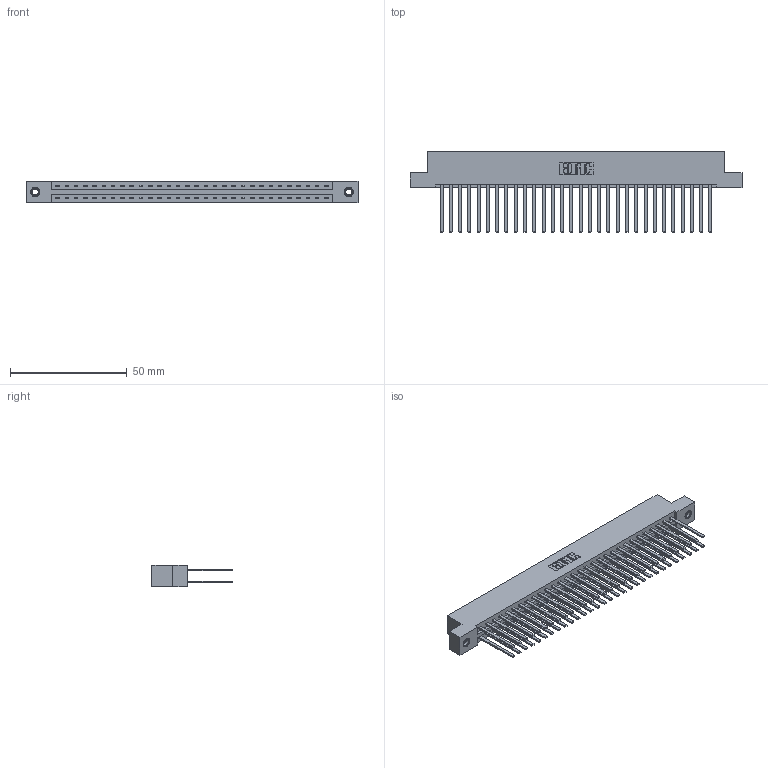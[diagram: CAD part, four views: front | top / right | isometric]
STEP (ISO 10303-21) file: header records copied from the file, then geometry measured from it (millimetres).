
FILE_DESCRIPTION (( 'STEP AP203' ), '1' );
FILE_NAME ('387-060-544-207.STEP', '2019-10-19T13:50:21', ( '' ), ( '' ), 'SwSTEP 2.0', 'SolidWorks 2016', '' );
FILE_SCHEMA (( 'CONFIG_CONTROL_DESIGN' ));
Length unit declared in the file: inch
Products named in the file (4): 345-292-001_345-293-144; 387-060-544-207; 345-250-001_345-250-005-103; 337 Part_Flush Mounting Lugs - 0.156 Dia-TI
Assembly tree (63 placements, depth 2):
  387-060-544-207
    337 Part_Flush Mounting Lugs - 0.156 Dia-TI
    345-292-001_345-293-144  x60
    345-250-001_345-250-005-103  x2
Bounding box: 141.88 x 34.3 x 9.4 mm (x, y, z)
Volume: 15620.7 mm3; surface area: 20326.3 mm2
Topology: 63 solids, 63 shells, 3054 faces, 9027 edges, 5930 vertices
Faces by surface type: plane 2142, cylinder 896, cone 12, torus 4
Entity records: 25814 total; most frequent: CARTESIAN_POINT 4337, ORIENTED_EDGE 4266, DIRECTION 3739, EDGE_CURVE 2133, LINE 1989, VECTOR 1989, VERTEX_POINT 1416, AXIS2_PLACEMENT_3D 875
